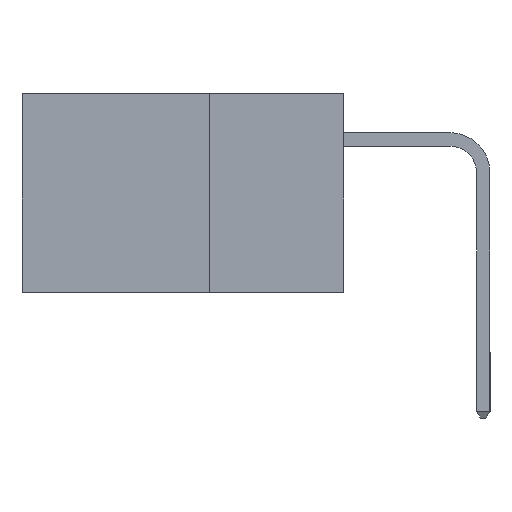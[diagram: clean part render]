
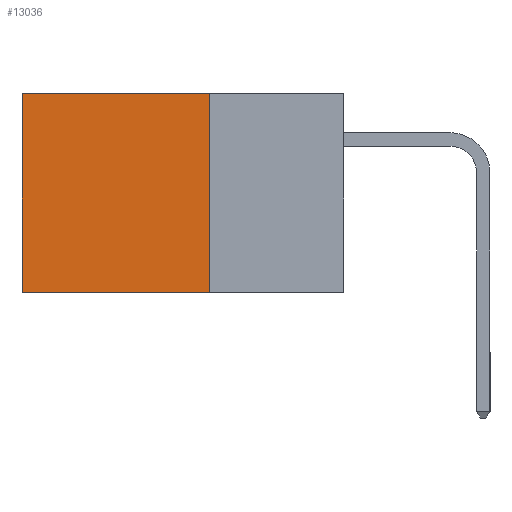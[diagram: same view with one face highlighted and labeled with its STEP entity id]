
A CAD part, left-side view. The second image highlights one B-rep face of the part: STEP entity #13036.
In plain terms, the highlighted planar face has unit normal (-1, 0, 0).
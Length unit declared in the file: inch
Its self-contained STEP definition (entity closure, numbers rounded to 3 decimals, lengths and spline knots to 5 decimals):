
#258 = CARTESIAN_POINT ( 'NONE',  ( 0.298, 0.6, -0.37 ) ) ;
#1155 = DIRECTION ( 'NONE',  ( 0., 1., 0. ) ) ;
#2014 = CARTESIAN_POINT ( 'NONE',  ( 0.298, 0.25, 0. ) ) ;
#2067 = DIRECTION ( 'NONE',  ( 0., 0., -1. ) ) ;
#2477 = EDGE_CURVE ( 'NONE', #3346, #5030, #13007, .T. ) ;
#2514 = CARTESIAN_POINT ( 'NONE',  ( 0.298, 0.25, 0. ) ) ;
#2728 = FACE_OUTER_BOUND ( 'NONE', #6812, .T. ) ;
#2951 = CARTESIAN_POINT ( 'NONE',  ( 0.298, 0.25, -0.37 ) ) ;
#3145 = VERTEX_POINT ( 'NONE', #258 ) ;
#3346 = VERTEX_POINT ( 'NONE', #3991 ) ;
#3478 = DIRECTION ( 'NONE',  ( 0., 0., -1. ) ) ;
#3705 = ORIENTED_EDGE ( 'NONE', *, *, #8837, .F. ) ;
#3795 = PLANE ( 'NONE',  #12271 ) ;
#3991 = CARTESIAN_POINT ( 'NONE',  ( 0.298, 0.25, 0. ) ) ;
#4118 = CARTESIAN_POINT ( 'NONE',  ( 0.298, 0.6, 0. ) ) ;
#4247 = EDGE_CURVE ( 'NONE', #5030, #3145, #13279, .T. ) ;
#4779 = ORIENTED_EDGE ( 'NONE', *, *, #2477, .T. ) ;
#5030 = VERTEX_POINT ( 'NONE', #4118 ) ;
#5656 = DIRECTION ( 'NONE',  ( 0., 1., 0. ) ) ;
#6282 = EDGE_CURVE ( 'NONE', #3346, #9928, #9499, .T. ) ;
#6812 = EDGE_LOOP ( 'NONE', ( #13524, #3705, #13638, #4779 ) ) ;
#8378 = CARTESIAN_POINT ( 'NONE',  ( 0.298, 0.25, 0. ) ) ;
#8837 = EDGE_CURVE ( 'NONE', #9928, #3145, #8847, .T. ) ;
#8847 = LINE ( 'NONE', #15133, #11642 ) ;
#9499 = LINE ( 'NONE', #2014, #10074 ) ;
#9928 = VERTEX_POINT ( 'NONE', #2951 ) ;
#10074 = VECTOR ( 'NONE', #2067, 39.37008 ) ;
#10545 = CARTESIAN_POINT ( 'NONE',  ( 0.298, 0.6, 0. ) ) ;
#11642 = VECTOR ( 'NONE', #5656, 39.37008 ) ;
#11783 = VECTOR ( 'NONE', #3478, 39.37008 ) ;
#11957 = DIRECTION ( 'NONE',  ( 1., 0., 0. ) ) ;
#12271 = AXIS2_PLACEMENT_3D ( 'NONE', #8378, #11957, #13164 ) ;
#13007 = LINE ( 'NONE', #2514, #14458 ) ;
#13036 = ADVANCED_FACE ( 'NONE', ( #2728 ), #3795, .F. ) ;
#13164 = DIRECTION ( 'NONE',  ( 0., 0., -1. ) ) ;
#13279 = LINE ( 'NONE', #10545, #11783 ) ;
#13524 = ORIENTED_EDGE ( 'NONE', *, *, #4247, .T. ) ;
#13638 = ORIENTED_EDGE ( 'NONE', *, *, #6282, .F. ) ;
#14458 = VECTOR ( 'NONE', #1155, 39.37008 ) ;
#15133 = CARTESIAN_POINT ( 'NONE',  ( 0.298, 0.25, -0.37 ) ) ;
